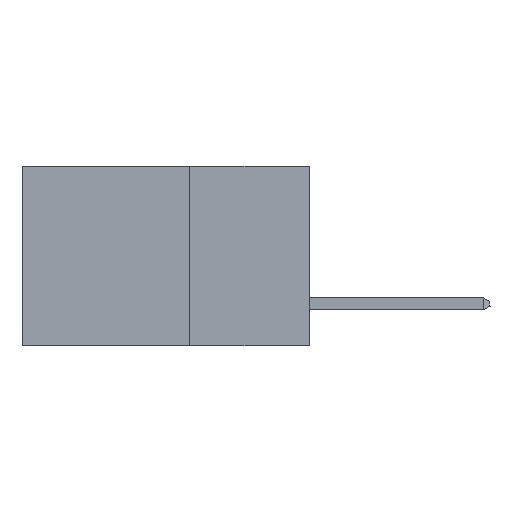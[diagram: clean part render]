
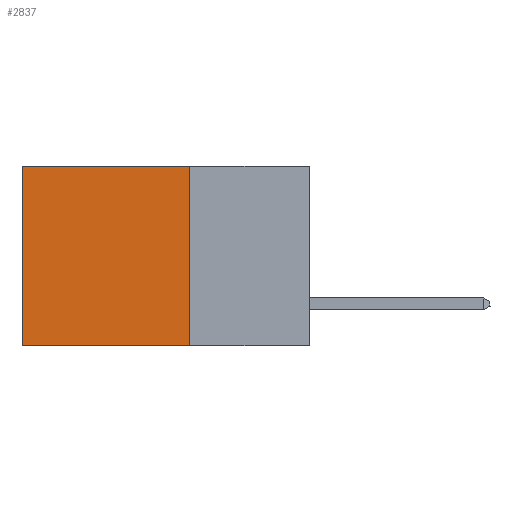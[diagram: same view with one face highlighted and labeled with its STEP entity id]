
A CAD part, left-side view. The second image highlights one B-rep face of the part: STEP entity #2837.
In plain terms, the highlighted planar face has unit normal (-1, 0, 0).
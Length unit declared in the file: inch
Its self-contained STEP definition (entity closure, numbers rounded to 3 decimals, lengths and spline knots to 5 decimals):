
#352 = CARTESIAN_POINT ( 'NONE',  ( 0.2875, 0.25, -0.375 ) ) ;
#449 = VECTOR ( 'NONE', #969, 39.37008 ) ;
#969 = DIRECTION ( 'NONE',  ( 0., 1., 0. ) ) ;
#1109 = LINE ( 'NONE', #17440, #14453 ) ;
#1908 = VERTEX_POINT ( 'NONE', #13233 ) ;
#1921 = EDGE_CURVE ( 'NONE', #20792, #1908, #15506, .T. ) ;
#2432 = CARTESIAN_POINT ( 'NONE',  ( 0.2875, 0.25, 0. ) ) ;
#2778 = DIRECTION ( 'NONE',  ( 0., 0., -1. ) ) ;
#2837 = ADVANCED_FACE ( 'NONE', ( #14724 ), #17657, .F. ) ;
#3443 = DIRECTION ( 'NONE',  ( 0., 0., -1. ) ) ;
#3684 = CARTESIAN_POINT ( 'NONE',  ( 0.2875, 0.25, -0.375 ) ) ;
#5868 = CARTESIAN_POINT ( 'NONE',  ( 0.2875, 0.6, 0. ) ) ;
#7191 = ORIENTED_EDGE ( 'NONE', *, *, #16671, .T. ) ;
#8011 = DIRECTION ( 'NONE',  ( 0., 0., -1. ) ) ;
#10460 = VECTOR ( 'NONE', #3443, 39.37008 ) ;
#12211 = EDGE_CURVE ( 'NONE', #20792, #18681, #13777, .T. ) ;
#12424 = CARTESIAN_POINT ( 'NONE',  ( 0.2875, 0.25, 0. ) ) ;
#12793 = VERTEX_POINT ( 'NONE', #13951 ) ;
#13105 = ORIENTED_EDGE ( 'NONE', *, *, #12211, .T. ) ;
#13233 = CARTESIAN_POINT ( 'NONE',  ( 0.2875, 0.25, -0.375 ) ) ;
#13777 = LINE ( 'NONE', #12424, #449 ) ;
#13951 = CARTESIAN_POINT ( 'NONE',  ( 0.2875, 0.6, -0.375 ) ) ;
#14289 = DIRECTION ( 'NONE',  ( 1., 0., 0. ) ) ;
#14453 = VECTOR ( 'NONE', #2778, 39.37008 ) ;
#14599 = AXIS2_PLACEMENT_3D ( 'NONE', #15847, #14289, #8011 ) ;
#14724 = FACE_OUTER_BOUND ( 'NONE', #18951, .T. ) ;
#14744 = ORIENTED_EDGE ( 'NONE', *, *, #16177, .F. ) ;
#14753 = VECTOR ( 'NONE', #16625, 39.37008 ) ;
#15506 = LINE ( 'NONE', #352, #10460 ) ;
#15847 = CARTESIAN_POINT ( 'NONE',  ( 0.2875, 0.25, -0.375 ) ) ;
#16177 = EDGE_CURVE ( 'NONE', #1908, #12793, #17752, .T. ) ;
#16625 = DIRECTION ( 'NONE',  ( 0., 1., 0. ) ) ;
#16671 = EDGE_CURVE ( 'NONE', #18681, #12793, #1109, .T. ) ;
#17169 = ORIENTED_EDGE ( 'NONE', *, *, #1921, .F. ) ;
#17440 = CARTESIAN_POINT ( 'NONE',  ( 0.2875, 0.6, -0.375 ) ) ;
#17657 = PLANE ( 'NONE',  #14599 ) ;
#17752 = LINE ( 'NONE', #3684, #14753 ) ;
#18681 = VERTEX_POINT ( 'NONE', #5868 ) ;
#18951 = EDGE_LOOP ( 'NONE', ( #7191, #14744, #17169, #13105 ) ) ;
#20792 = VERTEX_POINT ( 'NONE', #2432 ) ;
